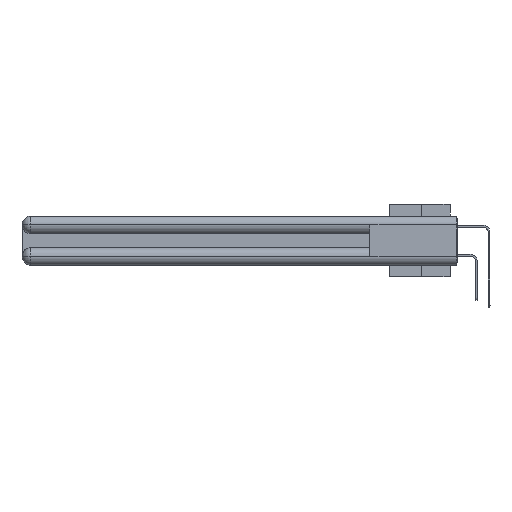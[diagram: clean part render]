
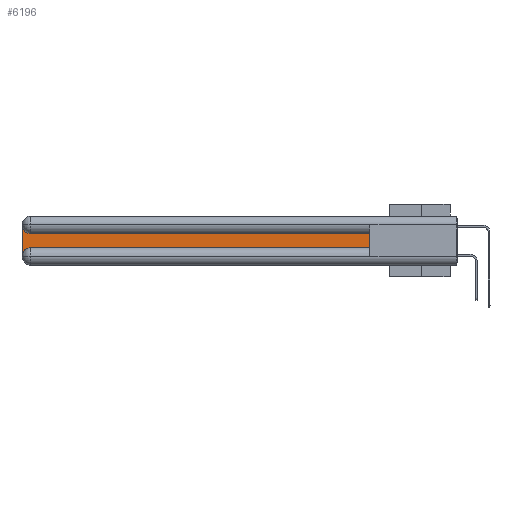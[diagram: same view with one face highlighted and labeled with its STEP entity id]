
A CAD part, left-side view. The second image highlights one B-rep face of the part: STEP entity #6196.
In plain terms, the highlighted planar face has unit normal (-1, 0, 0).
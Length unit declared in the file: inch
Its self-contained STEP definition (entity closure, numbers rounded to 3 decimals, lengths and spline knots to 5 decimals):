
#216 = DIRECTION ( 'NONE',  ( 0., 0., 1. ) ) ;
#2078 = DIRECTION ( 'NONE',  ( 0., -1., 0. ) ) ;
#2112 = CARTESIAN_POINT ( 'NONE',  ( 0.075, 2.94, -0.1225 ) ) ;
#3019 = CARTESIAN_POINT ( 'NONE',  ( 0.075, 3., -0.2775 ) ) ;
#3724 = VECTOR ( 'NONE', #2078, 39.37008 ) ;
#3841 = EDGE_CURVE ( 'NONE', #6055, #25682, #25783, .T. ) ;
#4124 = VERTEX_POINT ( 'NONE', #2112 ) ;
#4559 = EDGE_CURVE ( 'NONE', #25682, #9773, #25979, .T. ) ;
#5465 = DIRECTION ( 'NONE',  ( 1., 0., 0. ) ) ;
#5785 = CARTESIAN_POINT ( 'NONE',  ( 0.075, 2.94, -0.2775 ) ) ;
#6023 = CARTESIAN_POINT ( 'NONE',  ( 0.075, 3., -0.1225 ) ) ;
#6055 = VERTEX_POINT ( 'NONE', #3019 ) ;
#6196 = ADVANCED_FACE ( 'NONE', ( #25159 ), #25629, .F. ) ;
#6981 = ORIENTED_EDGE ( 'NONE', *, *, #24119, .T. ) ;
#7941 = VECTOR ( 'NONE', #21397, 39.37008 ) ;
#9773 = VERTEX_POINT ( 'NONE', #15040 ) ;
#10690 = CARTESIAN_POINT ( 'NONE',  ( 0.075, 0.6, -0.2175 ) ) ;
#11107 = DIRECTION ( 'NONE',  ( 1., 0., 0. ) ) ;
#11284 = EDGE_LOOP ( 'NONE', ( #19913, #13385, #6981, #26905, #30388, #21483 ) ) ;
#12324 = LINE ( 'NONE', #10690, #22790 ) ;
#13385 = ORIENTED_EDGE ( 'NONE', *, *, #21225, .T. ) ;
#13865 = CARTESIAN_POINT ( 'NONE',  ( 0.075, 0.6, -0.2175 ) ) ;
#13868 = LINE ( 'NONE', #21816, #30491 ) ;
#13897 = AXIS2_PLACEMENT_3D ( 'NONE', #6023, #11107, #27713 ) ;
#15040 = CARTESIAN_POINT ( 'NONE',  ( 0.075, 0.6, -0.2175 ) ) ;
#16790 = DIRECTION ( 'NONE',  ( 1., 0., 0. ) ) ;
#19817 = DIRECTION ( 'NONE',  ( 0., 0., -1. ) ) ;
#19913 = ORIENTED_EDGE ( 'NONE', *, *, #26872, .T. ) ;
#20639 = VERTEX_POINT ( 'NONE', #28486 ) ;
#20897 = VERTEX_POINT ( 'NONE', #24635 ) ;
#21020 = CARTESIAN_POINT ( 'NONE',  ( 0.075, 2.94, -0.2175 ) ) ;
#21225 = EDGE_CURVE ( 'NONE', #4124, #20639, #25194, .T. ) ;
#21397 = DIRECTION ( 'NONE',  ( 0., 0., -1. ) ) ;
#21483 = ORIENTED_EDGE ( 'NONE', *, *, #29794, .T. ) ;
#21547 = CARTESIAN_POINT ( 'NONE',  ( 0.075, 3., -0.2175 ) ) ;
#21816 = CARTESIAN_POINT ( 'NONE',  ( 0.075, 0.6, -0.1225 ) ) ;
#22790 = VECTOR ( 'NONE', #216, 39.37008 ) ;
#23980 = CARTESIAN_POINT ( 'NONE',  ( 0.075, 2.94, -0.0625 ) ) ;
#24119 = EDGE_CURVE ( 'NONE', #20639, #6055, #28417, .T. ) ;
#24635 = CARTESIAN_POINT ( 'NONE',  ( 0.075, 0.6, -0.1225 ) ) ;
#25159 = FACE_OUTER_BOUND ( 'NONE', #11284, .T. ) ;
#25194 = CIRCLE ( 'NONE', #28749, 0.06 ) ;
#25260 = AXIS2_PLACEMENT_3D ( 'NONE', #5785, #5465, #27627 ) ;
#25629 = PLANE ( 'NONE',  #13897 ) ;
#25682 = VERTEX_POINT ( 'NONE', #21020 ) ;
#25783 = CIRCLE ( 'NONE', #25260, 0.06 ) ;
#25979 = LINE ( 'NONE', #13865, #3724 ) ;
#26442 = DIRECTION ( 'NONE',  ( 0., 1., 0. ) ) ;
#26872 = EDGE_CURVE ( 'NONE', #20897, #4124, #13868, .T. ) ;
#26905 = ORIENTED_EDGE ( 'NONE', *, *, #3841, .T. ) ;
#27627 = DIRECTION ( 'NONE',  ( 0., 0., -1. ) ) ;
#27713 = DIRECTION ( 'NONE',  ( 0., 0., -1. ) ) ;
#28417 = LINE ( 'NONE', #21547, #7941 ) ;
#28486 = CARTESIAN_POINT ( 'NONE',  ( 0.075, 3., -0.0625 ) ) ;
#28749 = AXIS2_PLACEMENT_3D ( 'NONE', #23980, #16790, #19817 ) ;
#29794 = EDGE_CURVE ( 'NONE', #9773, #20897, #12324, .T. ) ;
#30388 = ORIENTED_EDGE ( 'NONE', *, *, #4559, .T. ) ;
#30491 = VECTOR ( 'NONE', #26442, 39.37008 ) ;
